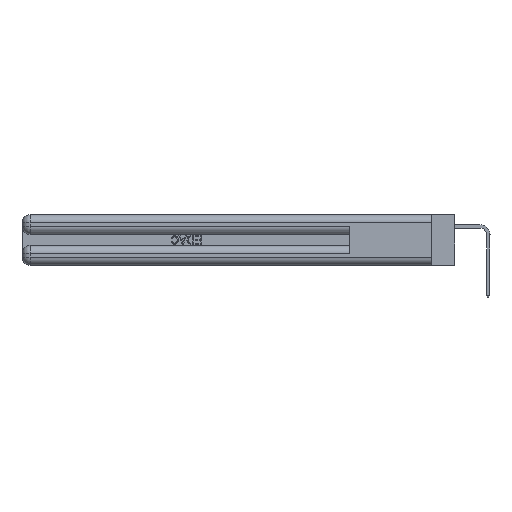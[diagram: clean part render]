
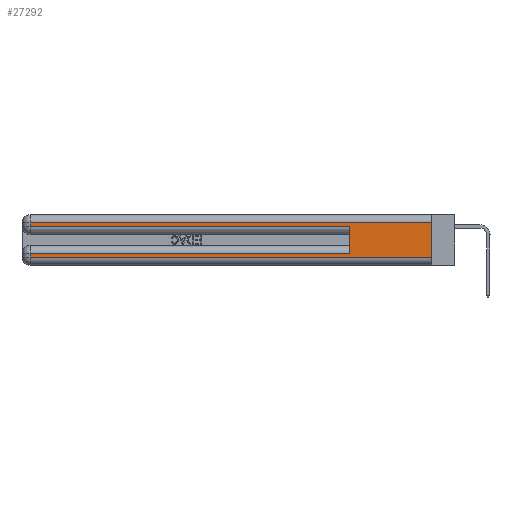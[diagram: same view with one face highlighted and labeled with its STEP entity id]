
A CAD part, left-side view. The second image highlights one B-rep face of the part: STEP entity #27292.
In plain terms, the highlighted planar face has unit normal (-1, 0, 0).
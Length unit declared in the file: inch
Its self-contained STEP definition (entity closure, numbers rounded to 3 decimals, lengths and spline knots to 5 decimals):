
#1721 = VERTEX_POINT ( 'NONE', #8315 ) ;
#2502 = VECTOR ( 'NONE', #13627, 39.37008 ) ;
#2503 = ORIENTED_EDGE ( 'NONE', *, *, #34336, .T. ) ;
#2949 = VERTEX_POINT ( 'NONE', #12853 ) ;
#3987 = ORIENTED_EDGE ( 'NONE', *, *, #9954, .F. ) ;
#4582 = PLANE ( 'NONE',  #32786 ) ;
#5000 = DIRECTION ( 'NONE',  ( 0., 0., -1. ) ) ;
#5021 = CARTESIAN_POINT ( 'NONE',  ( 0., 2.94, 0.37 ) ) ;
#7030 = DIRECTION ( 'NONE',  ( 0., 1., 0. ) ) ;
#7333 = CARTESIAN_POINT ( 'NONE',  ( 0., 2.94, 0.285 ) ) ;
#7395 = DIRECTION ( 'NONE',  ( 0., 0., 1. ) ) ;
#7489 = VECTOR ( 'NONE', #36031, 39.37008 ) ;
#8152 = DIRECTION ( 'NONE',  ( 0., 0., -1. ) ) ;
#8315 = CARTESIAN_POINT ( 'NONE',  ( 0., 2.94, 0.085 ) ) ;
#8909 = EDGE_LOOP ( 'NONE', ( #23172, #12659, #2503, #31314, #3987, #28863, #33092, #23063 ) ) ;
#9888 = VERTEX_POINT ( 'NONE', #10116 ) ;
#9954 = EDGE_CURVE ( 'NONE', #2949, #9888, #11207, .T. ) ;
#10116 = CARTESIAN_POINT ( 'NONE',  ( 0., 0.6, 0.285 ) ) ;
#10149 = VECTOR ( 'NONE', #7030, 39.37008 ) ;
#10776 = LINE ( 'NONE', #26134, #2502 ) ;
#10844 = DIRECTION ( 'NONE',  ( 0., 0., -1. ) ) ;
#11149 = LINE ( 'NONE', #13186, #10149 ) ;
#11207 = LINE ( 'NONE', #23029, #34416 ) ;
#12206 = VERTEX_POINT ( 'NONE', #15976 ) ;
#12520 = EDGE_CURVE ( 'NONE', #12206, #31132, #21867, .T. ) ;
#12659 = ORIENTED_EDGE ( 'NONE', *, *, #28657, .T. ) ;
#12735 = CARTESIAN_POINT ( 'NONE',  ( 0., 2.94, 0.37 ) ) ;
#12853 = CARTESIAN_POINT ( 'NONE',  ( 0., 0.6, 0.085 ) ) ;
#13186 = CARTESIAN_POINT ( 'NONE',  ( 0., 0., 0.31 ) ) ;
#13627 = DIRECTION ( 'NONE',  ( 0., -1., 0. ) ) ;
#13966 = VECTOR ( 'NONE', #31769, 39.37008 ) ;
#15976 = CARTESIAN_POINT ( 'NONE',  ( 0., 0., 0.31 ) ) ;
#17123 = CARTESIAN_POINT ( 'NONE',  ( 0., 0., 0.085 ) ) ;
#17673 = EDGE_CURVE ( 'NONE', #2949, #1721, #24182, .T. ) ;
#19773 = EDGE_CURVE ( 'NONE', #31749, #31132, #10776, .T. ) ;
#19933 = EDGE_CURVE ( 'NONE', #1721, #31749, #29984, .T. ) ;
#20336 = CARTESIAN_POINT ( 'NONE',  ( 0., 2.94, 0.31 ) ) ;
#20789 = DIRECTION ( 'NONE',  ( 0., -1., 0. ) ) ;
#21867 = LINE ( 'NONE', #26926, #28259 ) ;
#23029 = CARTESIAN_POINT ( 'NONE',  ( 0., 0.6, 0.145 ) ) ;
#23063 = ORIENTED_EDGE ( 'NONE', *, *, #19773, .T. ) ;
#23172 = ORIENTED_EDGE ( 'NONE', *, *, #12520, .F. ) ;
#24182 = LINE ( 'NONE', #17123, #7489 ) ;
#25249 = VECTOR ( 'NONE', #20789, 39.37008 ) ;
#25999 = FACE_OUTER_BOUND ( 'NONE', #8909, .T. ) ;
#26134 = CARTESIAN_POINT ( 'NONE',  ( 0., 0., 0.06 ) ) ;
#26501 = CARTESIAN_POINT ( 'NONE',  ( 0., 0., 0.37 ) ) ;
#26926 = CARTESIAN_POINT ( 'NONE',  ( 0., 0., 0.37 ) ) ;
#27292 = ADVANCED_FACE ( 'NONE', ( #25999 ), #4582, .F. ) ;
#28259 = VECTOR ( 'NONE', #5000, 39.37008 ) ;
#28657 = EDGE_CURVE ( 'NONE', #12206, #33264, #11149, .T. ) ;
#28863 = ORIENTED_EDGE ( 'NONE', *, *, #17673, .T. ) ;
#29708 = DIRECTION ( 'NONE',  ( 1., 0., 0. ) ) ;
#29984 = LINE ( 'NONE', #5021, #37410 ) ;
#31132 = VERTEX_POINT ( 'NONE', #37004 ) ;
#31314 = ORIENTED_EDGE ( 'NONE', *, *, #34728, .T. ) ;
#31749 = VERTEX_POINT ( 'NONE', #37642 ) ;
#31767 = LINE ( 'NONE', #12735, #13966 ) ;
#31769 = DIRECTION ( 'NONE',  ( 0., 0., -1. ) ) ;
#32786 = AXIS2_PLACEMENT_3D ( 'NONE', #26501, #29708, #10844 ) ;
#33092 = ORIENTED_EDGE ( 'NONE', *, *, #19933, .T. ) ;
#33176 = VERTEX_POINT ( 'NONE', #7333 ) ;
#33264 = VERTEX_POINT ( 'NONE', #20336 ) ;
#33725 = LINE ( 'NONE', #36567, #25249 ) ;
#34336 = EDGE_CURVE ( 'NONE', #33264, #33176, #31767, .T. ) ;
#34416 = VECTOR ( 'NONE', #7395, 39.37008 ) ;
#34728 = EDGE_CURVE ( 'NONE', #33176, #9888, #33725, .T. ) ;
#36031 = DIRECTION ( 'NONE',  ( 0., 1., 0. ) ) ;
#36567 = CARTESIAN_POINT ( 'NONE',  ( 0., 0., 0.285 ) ) ;
#37004 = CARTESIAN_POINT ( 'NONE',  ( 0., 0., 0.06 ) ) ;
#37410 = VECTOR ( 'NONE', #8152, 39.37008 ) ;
#37642 = CARTESIAN_POINT ( 'NONE',  ( 0., 2.94, 0.06 ) ) ;
